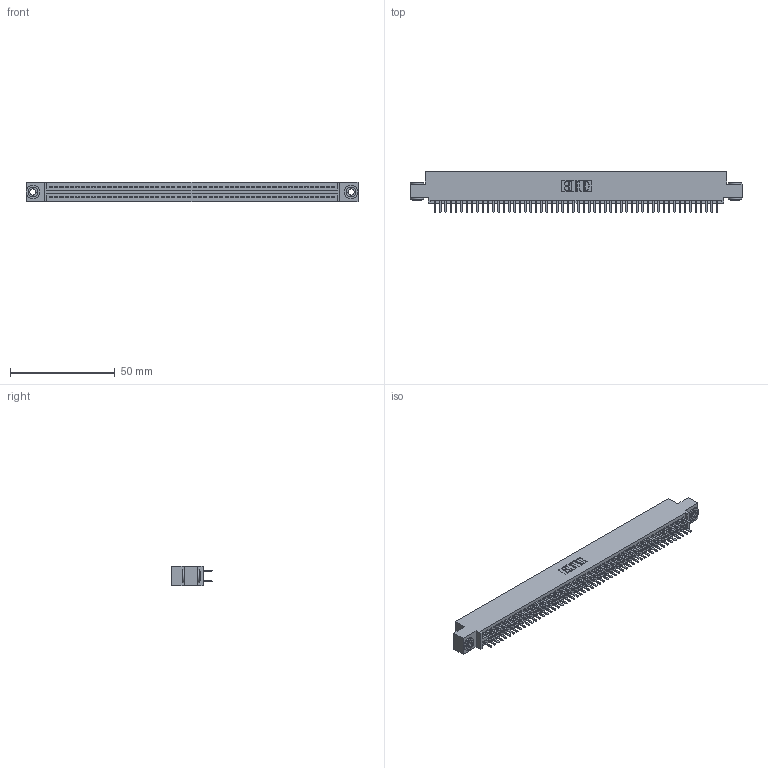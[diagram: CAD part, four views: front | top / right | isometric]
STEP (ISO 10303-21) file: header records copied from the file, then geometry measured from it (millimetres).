
FILE_DESCRIPTION (( 'STEP AP203' ), '1' );
FILE_NAME ('345-108-520-503.STEP', '2018-10-07T04:59:52', ( '' ), ( '' ), 'SwSTEP 2.0', 'SolidWorks 2016', '' );
FILE_SCHEMA (( 'CONFIG_CONTROL_DESIGN' ));
Length unit declared in the file: inch
Products named in the file (4): 345-108-520-503; 345 Part_0.110 Offset - 0.156 Dia-TH; 345-250-002_345-250-002-102; 345-292-001_345-293-120
Assembly tree (111 placements, depth 2):
  345-108-520-503
    345 Part_0.110 Offset - 0.156 Dia-TH
    345-292-001_345-293-120  x108
    345-250-002_345-250-002-102  x2
Bounding box: 158.37 x 19.68 x 9.4 mm (x, y, z)
Volume: 15394.1 mm3; surface area: 23184.2 mm2
Topology: 111 solids, 111 shells, 6000 faces, 17385 edges, 11298 vertices
Faces by surface type: plane 3874, cylinder 2118, cone 8
Entity records: 41650 total; most frequent: CARTESIAN_POINT 6959, ORIENTED_EDGE 6874, DIRECTION 6139, EDGE_CURVE 3437, LINE 3061, VECTOR 3061, VERTEX_POINT 2286, AXIS2_PLACEMENT_3D 1539
